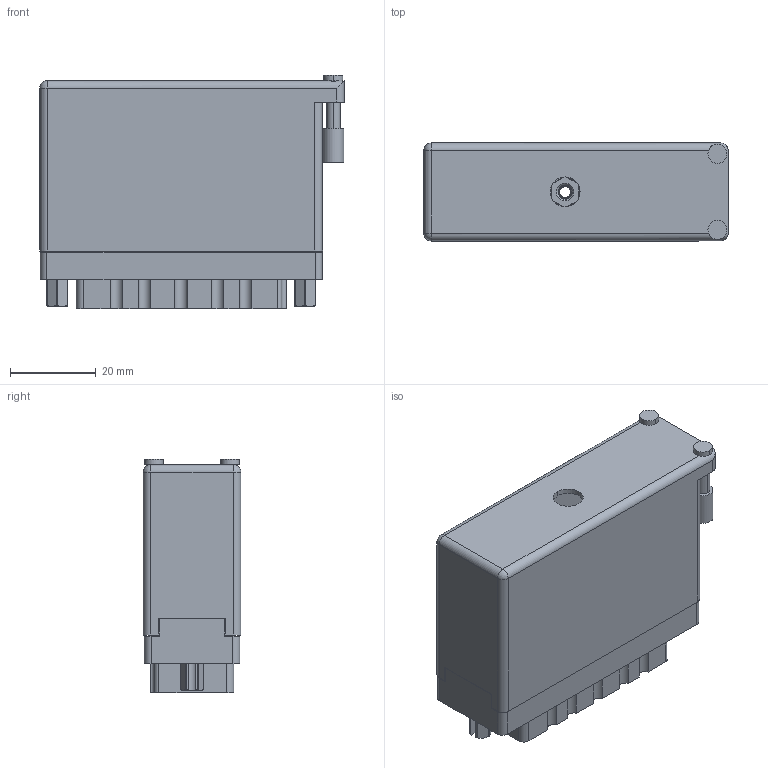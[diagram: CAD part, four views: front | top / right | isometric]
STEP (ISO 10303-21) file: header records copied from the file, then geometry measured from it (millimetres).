
FILE_DESCRIPTION (( 'STEP AP203' ), '1' );
FILE_NAME ('516-056-000-452.STEP', '2020-03-05T20:17:56', ( '' ), ( '' ), 'SwSTEP 2.0', 'SolidWorks 2016', '' );
FILE_SCHEMA (( 'CONFIG_CONTROL_DESIGN' ));
Length unit declared in the file: inch
Products named in the file (7): 516-056-000-452; 516-230-001_Metal - 056 Side Entry; 516-221-038-102_056; 516-221-038-102_057; 516-252-035-100_516-252-035-100; 516-252-021-102_056; 516 Part Receptacle_056
Assembly tree (7 placements, depth 2):
  516-056-000-452
    516 Part Receptacle_056
    516-230-001_Metal - 056 Side Entry
    516-252-021-102_056  x2
    516-221-038-102_056
    516-252-035-100_516-252-035-100
    516-221-038-102_057
Bounding box: 71.12 x 22.83 x 54.53 mm (x, y, z)
Volume: 25259 mm3; surface area: 37656.3 mm2
Topology: 7 solids, 7 shells, 1548 faces, 4499 edges, 2980 vertices
Faces by surface type: plane 984, cylinder 484, cone 44, bspline 34, sphere 2
Entity records: 57466 total; most frequent: CARTESIAN_POINT 15887, ORIENTED_EDGE 8806, DIRECTION 8331, EDGE_CURVE 4403, VECTOR 3035, LINE 3035, VERTEX_POINT 2920, AXIS2_PLACEMENT_3D 2648
